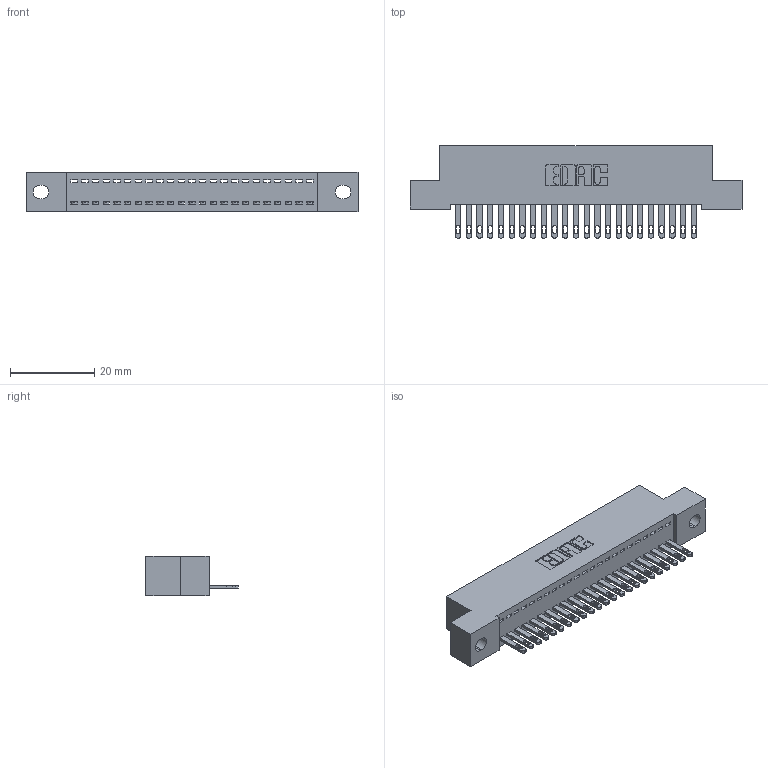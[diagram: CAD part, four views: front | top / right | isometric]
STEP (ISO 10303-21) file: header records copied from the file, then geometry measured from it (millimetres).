
FILE_DESCRIPTION (( 'STEP AP203' ), '1' );
FILE_NAME ('892-023-500-102.STEP', '2020-09-21T14:15:43', ( '' ), ( '' ), 'SwSTEP 2.0', 'SolidWorks 2020', '' );
FILE_SCHEMA (( 'CONFIG_CONTROL_DESIGN' ));
Length unit declared in the file: inch
Products named in the file (3): 345-292-001_345-293-100; 842 Part_.128 Slot; 892-023-500-102
Assembly tree (24 placements, depth 2):
  892-023-500-102
    842 Part_.128 Slot
    345-292-001_345-293-100  x23
Bounding box: 78.74 x 21.85 x 9.4 mm (x, y, z)
Volume: 6796 mm3; surface area: 9429.8 mm2
Topology: 24 solids, 24 shells, 1356 faces, 4175 edges, 2782 vertices
Faces by surface type: plane 898, cylinder 458
Entity records: 16451 total; most frequent: CARTESIAN_POINT 2847, ORIENTED_EDGE 2806, DIRECTION 2441, EDGE_CURVE 1403, LINE 1271, VECTOR 1271, VERTEX_POINT 934, AXIS2_PLACEMENT_3D 585
